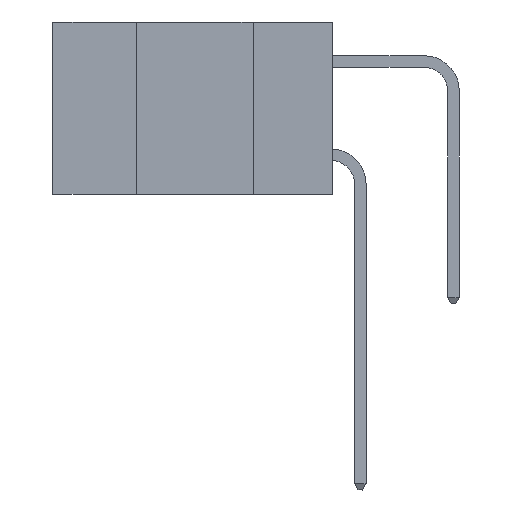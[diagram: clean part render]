
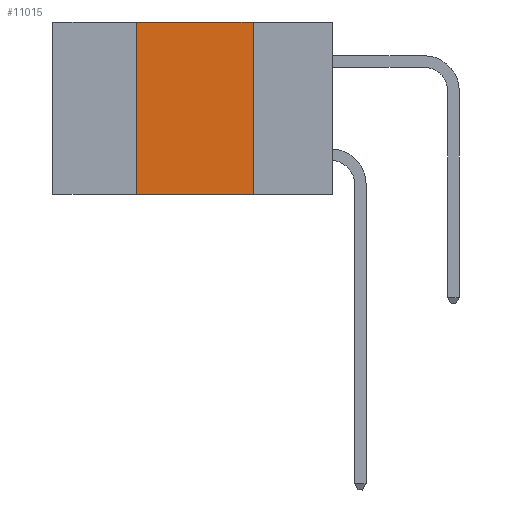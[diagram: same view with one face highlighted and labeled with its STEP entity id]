
A CAD part, left-side view. The second image highlights one B-rep face of the part: STEP entity #11015.
In plain terms, the highlighted planar face has unit normal (-1, 0, 0).
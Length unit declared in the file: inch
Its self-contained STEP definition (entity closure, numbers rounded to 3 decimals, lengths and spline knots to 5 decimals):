
#868 = CARTESIAN_POINT ( 'NONE',  ( 0., 0.42, 0. ) ) ;
#1175 = VECTOR ( 'NONE', #4740, 39.37008 ) ;
#1352 = CARTESIAN_POINT ( 'NONE',  ( 0., 0.17, 0. ) ) ;
#1438 = DIRECTION ( 'NONE',  ( 1., 0., 0. ) ) ;
#2113 = ORIENTED_EDGE ( 'NONE', *, *, #10553, .T. ) ;
#2504 = CARTESIAN_POINT ( 'NONE',  ( 0., 0.6, 0. ) ) ;
#2678 = CARTESIAN_POINT ( 'NONE',  ( 0., 0.42, -0.37 ) ) ;
#3608 = CARTESIAN_POINT ( 'NONE',  ( 0., 0.17, 0. ) ) ;
#4107 = ORIENTED_EDGE ( 'NONE', *, *, #6472, .F. ) ;
#4740 = DIRECTION ( 'NONE',  ( 0., -1., 0. ) ) ;
#4847 = ORIENTED_EDGE ( 'NONE', *, *, #8110, .F. ) ;
#5517 = VECTOR ( 'NONE', #5535, 39.37008 ) ;
#5535 = DIRECTION ( 'NONE',  ( 0., 0., -1. ) ) ;
#5652 = LINE ( 'NONE', #13143, #11626 ) ;
#6369 = EDGE_CURVE ( 'NONE', #13776, #14717, #13642, .T. ) ;
#6472 = EDGE_CURVE ( 'NONE', #14717, #9824, #14852, .T. ) ;
#6818 = VERTEX_POINT ( 'NONE', #2678 ) ;
#7152 = EDGE_LOOP ( 'NONE', ( #4107, #7592, #4847, #2113 ) ) ;
#7244 = PLANE ( 'NONE',  #10593 ) ;
#7580 = CARTESIAN_POINT ( 'NONE',  ( 0., 0.17, -0.37 ) ) ;
#7592 = ORIENTED_EDGE ( 'NONE', *, *, #6369, .F. ) ;
#7719 = DIRECTION ( 'NONE',  ( 0., -1., 0. ) ) ;
#7893 = LINE ( 'NONE', #11261, #13754 ) ;
#8110 = EDGE_CURVE ( 'NONE', #6818, #13776, #5652, .T. ) ;
#9699 = DIRECTION ( 'NONE',  ( 0., 0., -1. ) ) ;
#9824 = VERTEX_POINT ( 'NONE', #7580 ) ;
#10553 = EDGE_CURVE ( 'NONE', #6818, #9824, #7893, .T. ) ;
#10593 = AXIS2_PLACEMENT_3D ( 'NONE', #14295, #1438, #9699 ) ;
#11015 = ADVANCED_FACE ( 'NONE', ( #14331 ), #7244, .F. ) ;
#11261 = CARTESIAN_POINT ( 'NONE',  ( 0., 0.6, -0.37 ) ) ;
#11626 = VECTOR ( 'NONE', #13271, 39.37008 ) ;
#13143 = CARTESIAN_POINT ( 'NONE',  ( 0., 0.42, 0. ) ) ;
#13271 = DIRECTION ( 'NONE',  ( 0., 0., 1. ) ) ;
#13642 = LINE ( 'NONE', #2504, #1175 ) ;
#13754 = VECTOR ( 'NONE', #7719, 39.37008 ) ;
#13776 = VERTEX_POINT ( 'NONE', #868 ) ;
#14295 = CARTESIAN_POINT ( 'NONE',  ( 0., 0.6, 0. ) ) ;
#14331 = FACE_OUTER_BOUND ( 'NONE', #7152, .T. ) ;
#14717 = VERTEX_POINT ( 'NONE', #1352 ) ;
#14852 = LINE ( 'NONE', #3608, #5517 ) ;
